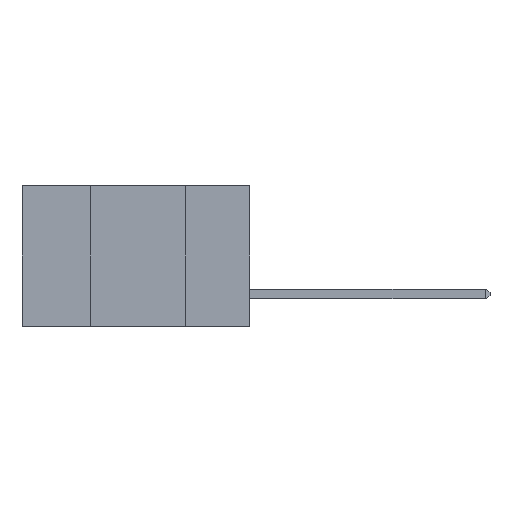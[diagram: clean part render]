
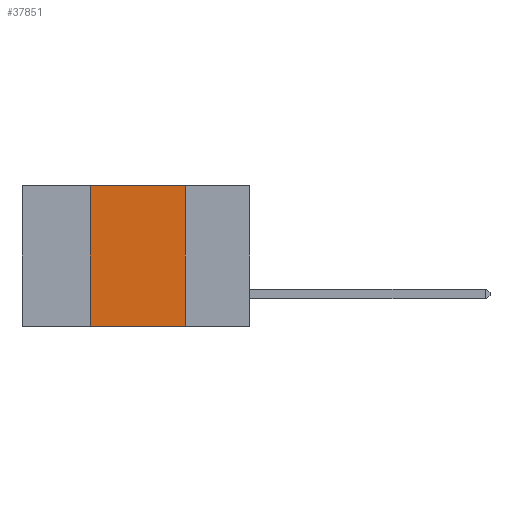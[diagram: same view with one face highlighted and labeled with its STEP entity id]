
A CAD part, left-side view. The second image highlights one B-rep face of the part: STEP entity #37851.
In plain terms, the highlighted planar face has unit normal (-1, 0, 0).
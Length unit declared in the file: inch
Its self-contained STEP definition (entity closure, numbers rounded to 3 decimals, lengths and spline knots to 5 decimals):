
#1335 = CARTESIAN_POINT ( 'NONE',  ( 0., 0.17, -0.37 ) ) ;
#4312 = DIRECTION ( 'NONE',  ( 0., 0., -1. ) ) ;
#5764 = VECTOR ( 'NONE', #23265, 39.37008 ) ;
#6701 = CARTESIAN_POINT ( 'NONE',  ( 0., 0.17, 0. ) ) ;
#7188 = ORIENTED_EDGE ( 'NONE', *, *, #26185, .F. ) ;
#8237 = LINE ( 'NONE', #26364, #15564 ) ;
#8696 = VECTOR ( 'NONE', #9842, 39.37008 ) ;
#8697 = EDGE_CURVE ( 'NONE', #25928, #17170, #18948, .T. ) ;
#9842 = DIRECTION ( 'NONE',  ( 0., 0., -1. ) ) ;
#13575 = PLANE ( 'NONE',  #19241 ) ;
#14033 = LINE ( 'NONE', #19995, #5764 ) ;
#15564 = VECTOR ( 'NONE', #16836, 39.37008 ) ;
#16836 = DIRECTION ( 'NONE',  ( 0., -1., 0. ) ) ;
#17043 = CARTESIAN_POINT ( 'NONE',  ( 0., 0.42, 0. ) ) ;
#17170 = VERTEX_POINT ( 'NONE', #1335 ) ;
#18520 = FACE_OUTER_BOUND ( 'NONE', #33521, .T. ) ;
#18666 = CARTESIAN_POINT ( 'NONE',  ( 0., 0.17, 0. ) ) ;
#18948 = LINE ( 'NONE', #6701, #8696 ) ;
#19241 = AXIS2_PLACEMENT_3D ( 'NONE', #35339, #22987, #4312 ) ;
#19995 = CARTESIAN_POINT ( 'NONE',  ( 0., 0.42, 0. ) ) ;
#22849 = CARTESIAN_POINT ( 'NONE',  ( 0., 0.6, 0. ) ) ;
#22987 = DIRECTION ( 'NONE',  ( 1., 0., 0. ) ) ;
#23265 = DIRECTION ( 'NONE',  ( 0., 0., 1. ) ) ;
#24888 = EDGE_CURVE ( 'NONE', #31594, #17170, #8237, .T. ) ;
#25715 = ORIENTED_EDGE ( 'NONE', *, *, #24888, .T. ) ;
#25827 = LINE ( 'NONE', #22849, #33132 ) ;
#25928 = VERTEX_POINT ( 'NONE', #18666 ) ;
#26185 = EDGE_CURVE ( 'NONE', #31594, #35430, #14033, .T. ) ;
#26364 = CARTESIAN_POINT ( 'NONE',  ( 0., 0.6, -0.37 ) ) ;
#27166 = ORIENTED_EDGE ( 'NONE', *, *, #8697, .F. ) ;
#31594 = VERTEX_POINT ( 'NONE', #34933 ) ;
#33132 = VECTOR ( 'NONE', #38483, 39.37008 ) ;
#33521 = EDGE_LOOP ( 'NONE', ( #27166, #36391, #7188, #25715 ) ) ;
#34933 = CARTESIAN_POINT ( 'NONE',  ( 0., 0.42, -0.37 ) ) ;
#35339 = CARTESIAN_POINT ( 'NONE',  ( 0., 0.6, 0. ) ) ;
#35430 = VERTEX_POINT ( 'NONE', #17043 ) ;
#36391 = ORIENTED_EDGE ( 'NONE', *, *, #37838, .F. ) ;
#37838 = EDGE_CURVE ( 'NONE', #35430, #25928, #25827, .T. ) ;
#37851 = ADVANCED_FACE ( 'NONE', ( #18520 ), #13575, .F. ) ;
#38483 = DIRECTION ( 'NONE',  ( 0., -1., 0. ) ) ;
